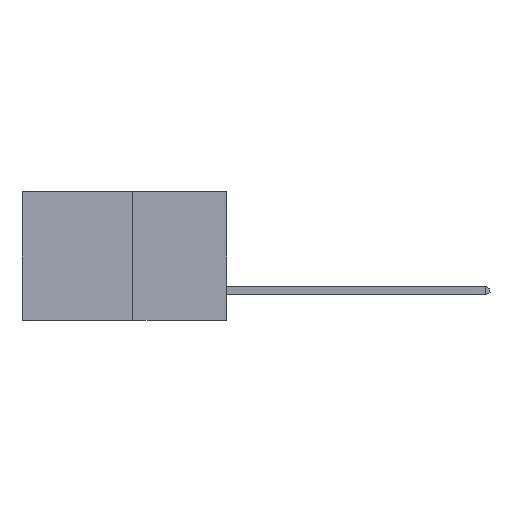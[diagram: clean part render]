
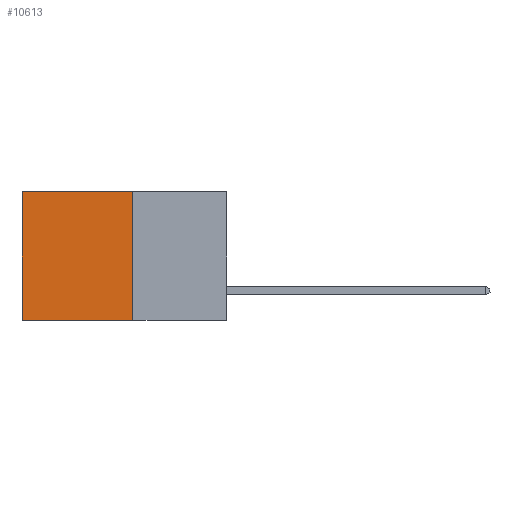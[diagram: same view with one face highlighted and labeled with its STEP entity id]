
A CAD part, left-side view. The second image highlights one B-rep face of the part: STEP entity #10613.
In plain terms, the highlighted planar face has unit normal (-1, 0, 0).
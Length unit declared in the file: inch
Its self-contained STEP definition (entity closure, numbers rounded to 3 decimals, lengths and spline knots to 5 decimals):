
#1048 = CARTESIAN_POINT ( 'NONE',  ( 0.277, 0.59, 0. ) ) ;
#1133 = VERTEX_POINT ( 'NONE', #12479 ) ;
#1621 = ORIENTED_EDGE ( 'NONE', *, *, #4491, .F. ) ;
#2098 = DIRECTION ( 'NONE',  ( 0., 1., 0. ) ) ;
#2508 = DIRECTION ( 'NONE',  ( 0., 0., -1. ) ) ;
#2789 = EDGE_LOOP ( 'NONE', ( #11107, #8848, #1621, #8774 ) ) ;
#3112 = FACE_OUTER_BOUND ( 'NONE', #2789, .T. ) ;
#3317 = DIRECTION ( 'NONE',  ( 0., 1., 0. ) ) ;
#3732 = DIRECTION ( 'NONE',  ( 1., 0., 0. ) ) ;
#4264 = VERTEX_POINT ( 'NONE', #11286 ) ;
#4474 = AXIS2_PLACEMENT_3D ( 'NONE', #11489, #3732, #10606 ) ;
#4491 = EDGE_CURVE ( 'NONE', #12567, #1133, #12407, .T. ) ;
#5566 = VERTEX_POINT ( 'NONE', #1048 ) ;
#5599 = VECTOR ( 'NONE', #2508, 39.37008 ) ;
#5737 = VECTOR ( 'NONE', #3317, 39.37008 ) ;
#7347 = EDGE_CURVE ( 'NONE', #12567, #5566, #10839, .T. ) ;
#7486 = VECTOR ( 'NONE', #9484, 39.37008 ) ;
#8101 = CARTESIAN_POINT ( 'NONE',  ( 0.277, 0.27, 0. ) ) ;
#8199 = LINE ( 'NONE', #9490, #5599 ) ;
#8587 = EDGE_CURVE ( 'NONE', #5566, #4264, #8199, .T. ) ;
#8774 = ORIENTED_EDGE ( 'NONE', *, *, #7347, .T. ) ;
#8848 = ORIENTED_EDGE ( 'NONE', *, *, #8949, .F. ) ;
#8949 = EDGE_CURVE ( 'NONE', #1133, #4264, #11558, .T. ) ;
#9481 = CARTESIAN_POINT ( 'NONE',  ( 0.277, 0.27, -0.37 ) ) ;
#9484 = DIRECTION ( 'NONE',  ( 0., 0., -1. ) ) ;
#9490 = CARTESIAN_POINT ( 'NONE',  ( 0.277, 0.59, -0.37 ) ) ;
#9682 = PLANE ( 'NONE',  #4474 ) ;
#10266 = CARTESIAN_POINT ( 'NONE',  ( 0.277, 0.27, 0. ) ) ;
#10606 = DIRECTION ( 'NONE',  ( 0., 0., -1. ) ) ;
#10613 = ADVANCED_FACE ( 'NONE', ( #3112 ), #9682, .F. ) ;
#10839 = LINE ( 'NONE', #10266, #5737 ) ;
#11107 = ORIENTED_EDGE ( 'NONE', *, *, #8587, .T. ) ;
#11270 = VECTOR ( 'NONE', #2098, 39.37008 ) ;
#11286 = CARTESIAN_POINT ( 'NONE',  ( 0.277, 0.59, -0.37 ) ) ;
#11489 = CARTESIAN_POINT ( 'NONE',  ( 0.277, 0.27, -0.37 ) ) ;
#11558 = LINE ( 'NONE', #11789, #11270 ) ;
#11789 = CARTESIAN_POINT ( 'NONE',  ( 0.277, 0.27, -0.37 ) ) ;
#12407 = LINE ( 'NONE', #9481, #7486 ) ;
#12479 = CARTESIAN_POINT ( 'NONE',  ( 0.277, 0.27, -0.37 ) ) ;
#12567 = VERTEX_POINT ( 'NONE', #8101 ) ;
